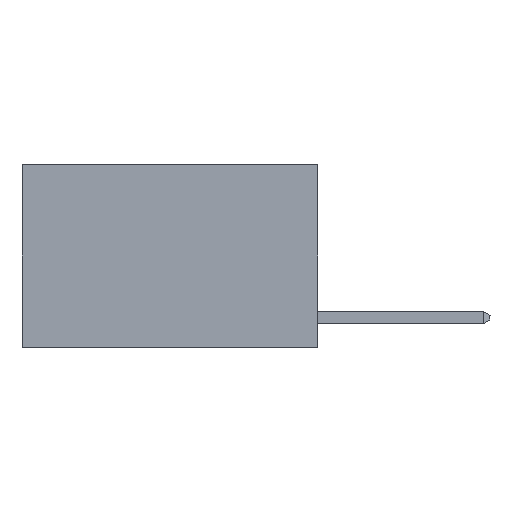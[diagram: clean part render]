
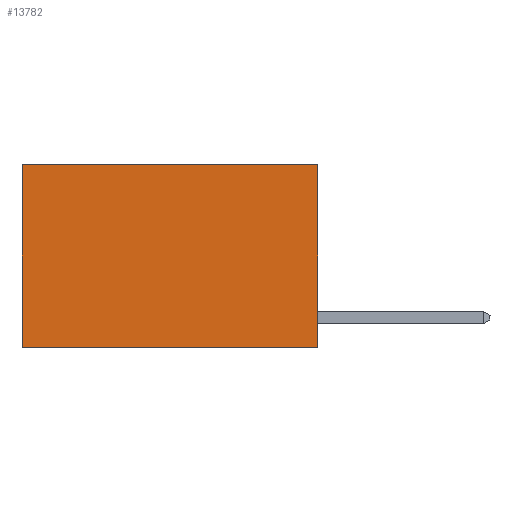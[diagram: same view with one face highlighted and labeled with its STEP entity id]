
A CAD part, left-side view. The second image highlights one B-rep face of the part: STEP entity #13782.
In plain terms, the highlighted planar face has unit normal (-1, 0, 0).
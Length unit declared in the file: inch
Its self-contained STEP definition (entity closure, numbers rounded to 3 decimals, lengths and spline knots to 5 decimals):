
#1125 = LINE ( 'NONE', #12493, #3905 ) ;
#1333 = DIRECTION ( 'NONE',  ( 0., 0., -1. ) ) ;
#1559 = CARTESIAN_POINT ( 'NONE',  ( 0.2625, 0.6, 0. ) ) ;
#1574 = EDGE_LOOP ( 'NONE', ( #16040, #23952, #20382, #17059 ) ) ;
#2855 = CARTESIAN_POINT ( 'NONE',  ( 0.2625, 0.6, -0.37 ) ) ;
#3772 = CARTESIAN_POINT ( 'NONE',  ( 0.2625, 0., 0. ) ) ;
#3905 = VECTOR ( 'NONE', #12244, 39.37008 ) ;
#5381 = LINE ( 'NONE', #3772, #23887 ) ;
#5540 = VECTOR ( 'NONE', #1333, 39.37008 ) ;
#7349 = LINE ( 'NONE', #22409, #17185 ) ;
#10435 = CARTESIAN_POINT ( 'NONE',  ( 0.2625, 0.6, 0. ) ) ;
#10934 = LINE ( 'NONE', #1559, #5540 ) ;
#11293 = DIRECTION ( 'NONE',  ( 0., 0., -1. ) ) ;
#12244 = DIRECTION ( 'NONE',  ( 0., 1., 0. ) ) ;
#12312 = EDGE_CURVE ( 'NONE', #15305, #15540, #7349, .T. ) ;
#12493 = CARTESIAN_POINT ( 'NONE',  ( 0.2625, 0., -0.37 ) ) ;
#13294 = VERTEX_POINT ( 'NONE', #23436 ) ;
#13782 = ADVANCED_FACE ( 'NONE', ( #19863 ), #17996, .F. ) ;
#14586 = CARTESIAN_POINT ( 'NONE',  ( 0.2625, 0., 0. ) ) ;
#15305 = VERTEX_POINT ( 'NONE', #14586 ) ;
#15540 = VERTEX_POINT ( 'NONE', #10435 ) ;
#16040 = ORIENTED_EDGE ( 'NONE', *, *, #23578, .T. ) ;
#16611 = CARTESIAN_POINT ( 'NONE',  ( 0.2625, 0., 0. ) ) ;
#17059 = ORIENTED_EDGE ( 'NONE', *, *, #12312, .T. ) ;
#17185 = VECTOR ( 'NONE', #20709, 39.37008 ) ;
#17996 = PLANE ( 'NONE',  #18803 ) ;
#18803 = AXIS2_PLACEMENT_3D ( 'NONE', #16611, #21699, #23524 ) ;
#19035 = EDGE_CURVE ( 'NONE', #15305, #13294, #5381, .T. ) ;
#19863 = FACE_OUTER_BOUND ( 'NONE', #1574, .T. ) ;
#20382 = ORIENTED_EDGE ( 'NONE', *, *, #19035, .F. ) ;
#20709 = DIRECTION ( 'NONE',  ( 0., 1., 0. ) ) ;
#21032 = EDGE_CURVE ( 'NONE', #13294, #21052, #1125, .T. ) ;
#21052 = VERTEX_POINT ( 'NONE', #2855 ) ;
#21699 = DIRECTION ( 'NONE',  ( 1., 0., 0. ) ) ;
#22409 = CARTESIAN_POINT ( 'NONE',  ( 0.2625, 0., 0. ) ) ;
#23436 = CARTESIAN_POINT ( 'NONE',  ( 0.2625, 0., -0.37 ) ) ;
#23524 = DIRECTION ( 'NONE',  ( 0., 0., -1. ) ) ;
#23578 = EDGE_CURVE ( 'NONE', #15540, #21052, #10934, .T. ) ;
#23887 = VECTOR ( 'NONE', #11293, 39.37008 ) ;
#23952 = ORIENTED_EDGE ( 'NONE', *, *, #21032, .F. ) ;
